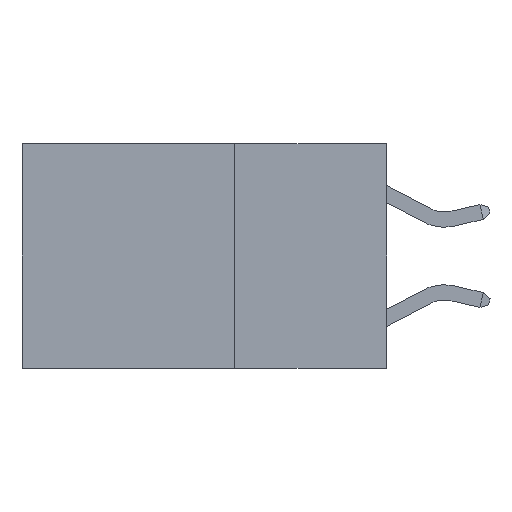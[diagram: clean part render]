
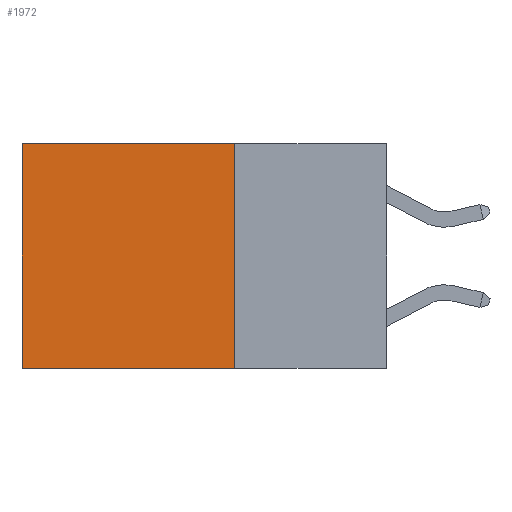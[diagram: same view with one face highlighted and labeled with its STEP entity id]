
A CAD part, left-side view. The second image highlights one B-rep face of the part: STEP entity #1972.
In plain terms, the highlighted planar face has unit normal (-1, 0, 0).
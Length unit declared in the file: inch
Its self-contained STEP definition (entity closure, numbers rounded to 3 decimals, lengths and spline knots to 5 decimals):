
#112 = DIRECTION ( 'NONE',  ( 0., 1., 0. ) ) ;
#609 = CARTESIAN_POINT ( 'NONE',  ( 0.2625, 0.6, -0.37 ) ) ;
#699 = FACE_OUTER_BOUND ( 'NONE', #7395, .T. ) ;
#1192 = VECTOR ( 'NONE', #7099, 39.37008 ) ;
#1972 = ADVANCED_FACE ( 'NONE', ( #699 ), #4172, .F. ) ;
#1983 = EDGE_CURVE ( 'NONE', #4372, #7480, #4477, .T. ) ;
#2149 = CARTESIAN_POINT ( 'NONE',  ( 0.2625, 0.6, 0. ) ) ;
#2952 = CARTESIAN_POINT ( 'NONE',  ( 0.2625, 0.25, -0.37 ) ) ;
#3018 = CARTESIAN_POINT ( 'NONE',  ( 0.2625, 0.25, 0. ) ) ;
#3194 = AXIS2_PLACEMENT_3D ( 'NONE', #3739, #3721, #4145 ) ;
#3200 = VECTOR ( 'NONE', #8134, 39.37008 ) ;
#3206 = DIRECTION ( 'NONE',  ( 0., 0., -1. ) ) ;
#3427 = VECTOR ( 'NONE', #112, 39.37008 ) ;
#3506 = CARTESIAN_POINT ( 'NONE',  ( 0.2625, 0.25, 0. ) ) ;
#3721 = DIRECTION ( 'NONE',  ( 1., 0., 0. ) ) ;
#3739 = CARTESIAN_POINT ( 'NONE',  ( 0.2625, 0.25, 0. ) ) ;
#3769 = VERTEX_POINT ( 'NONE', #2952 ) ;
#3781 = CARTESIAN_POINT ( 'NONE',  ( 0.2625, 0.25, 0. ) ) ;
#4145 = DIRECTION ( 'NONE',  ( 0., 0., -1. ) ) ;
#4172 = PLANE ( 'NONE',  #3194 ) ;
#4372 = VERTEX_POINT ( 'NONE', #2149 ) ;
#4434 = CARTESIAN_POINT ( 'NONE',  ( 0.2625, 0.6, 0. ) ) ;
#4477 = LINE ( 'NONE', #4434, #6036 ) ;
#4948 = LINE ( 'NONE', #3781, #1192 ) ;
#5238 = EDGE_CURVE ( 'NONE', #7636, #4372, #4948, .T. ) ;
#5343 = LINE ( 'NONE', #3506, #3200 ) ;
#5755 = ORIENTED_EDGE ( 'NONE', *, *, #1983, .T. ) ;
#5770 = EDGE_CURVE ( 'NONE', #7636, #3769, #5343, .T. ) ;
#6019 = ORIENTED_EDGE ( 'NONE', *, *, #7688, .F. ) ;
#6036 = VECTOR ( 'NONE', #3206, 39.37008 ) ;
#6666 = ORIENTED_EDGE ( 'NONE', *, *, #5770, .F. ) ;
#6704 = LINE ( 'NONE', #8311, #3427 ) ;
#7099 = DIRECTION ( 'NONE',  ( 0., 1., 0. ) ) ;
#7261 = ORIENTED_EDGE ( 'NONE', *, *, #5238, .T. ) ;
#7395 = EDGE_LOOP ( 'NONE', ( #5755, #6019, #6666, #7261 ) ) ;
#7480 = VERTEX_POINT ( 'NONE', #609 ) ;
#7636 = VERTEX_POINT ( 'NONE', #3018 ) ;
#7688 = EDGE_CURVE ( 'NONE', #3769, #7480, #6704, .T. ) ;
#8134 = DIRECTION ( 'NONE',  ( 0., 0., -1. ) ) ;
#8311 = CARTESIAN_POINT ( 'NONE',  ( 0.2625, 0.25, -0.37 ) ) ;
